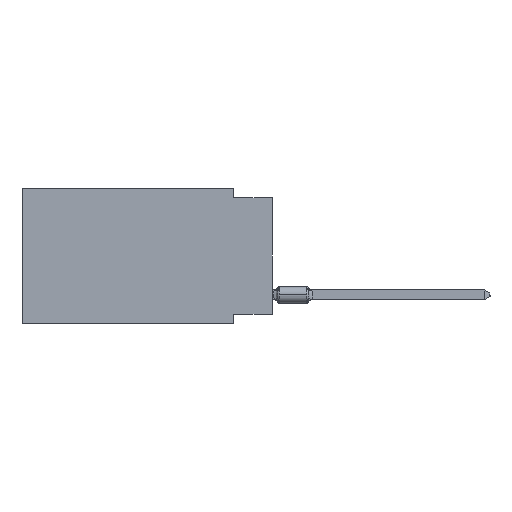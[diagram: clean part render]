
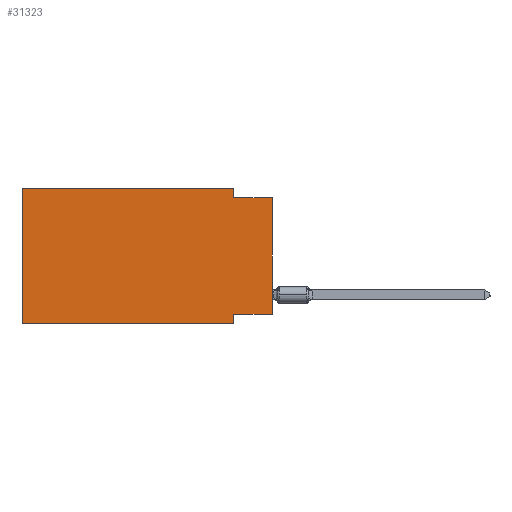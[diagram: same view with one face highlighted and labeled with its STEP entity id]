
A CAD part, left-side view. The second image highlights one B-rep face of the part: STEP entity #31323.
In plain terms, the highlighted planar face has unit normal (-1, 0, 0).
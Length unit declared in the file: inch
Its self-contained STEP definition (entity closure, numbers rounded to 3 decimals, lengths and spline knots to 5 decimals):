
#214 = LINE ( 'NONE', #24951, #24612 ) ;
#519 = VECTOR ( 'NONE', #20973, 39.37008 ) ;
#602 = VECTOR ( 'NONE', #39608, 39.37008 ) ;
#625 = VERTEX_POINT ( 'NONE', #37924 ) ;
#1147 = ORIENTED_EDGE ( 'NONE', *, *, #5059, .F. ) ;
#1822 = CARTESIAN_POINT ( 'NONE',  ( 0., 0.1, 0. ) ) ;
#1832 = CARTESIAN_POINT ( 'NONE',  ( 0., 0.645, -0.35 ) ) ;
#2816 = LINE ( 'NONE', #36383, #602 ) ;
#2853 = CARTESIAN_POINT ( 'NONE',  ( 0., 0., -0.325 ) ) ;
#3285 = ORIENTED_EDGE ( 'NONE', *, *, #30769, .T. ) ;
#5000 = ORIENTED_EDGE ( 'NONE', *, *, #15550, .F. ) ;
#5059 = EDGE_CURVE ( 'NONE', #625, #25514, #17745, .T. ) ;
#5633 = LINE ( 'NONE', #12036, #6264 ) ;
#6264 = VECTOR ( 'NONE', #36581, 39.37008 ) ;
#6781 = ORIENTED_EDGE ( 'NONE', *, *, #39465, .F. ) ;
#7541 = CARTESIAN_POINT ( 'NONE',  ( 0., 0.1, 0. ) ) ;
#7728 = DIRECTION ( 'NONE',  ( 0., -1., 0. ) ) ;
#7756 = CARTESIAN_POINT ( 'NONE',  ( 0., 0., -0.025 ) ) ;
#7968 = VECTOR ( 'NONE', #17562, 39.37008 ) ;
#9102 = EDGE_CURVE ( 'NONE', #15400, #625, #14931, .T. ) ;
#9304 = CARTESIAN_POINT ( 'NONE',  ( 0., 0.1, -0.35 ) ) ;
#10879 = AXIS2_PLACEMENT_3D ( 'NONE', #29014, #20142, #32430 ) ;
#11388 = VERTEX_POINT ( 'NONE', #15089 ) ;
#11724 = CARTESIAN_POINT ( 'NONE',  ( 0., 0., -0.325 ) ) ;
#12036 = CARTESIAN_POINT ( 'NONE',  ( 0., 0., -0.025 ) ) ;
#12928 = EDGE_CURVE ( 'NONE', #27492, #26486, #5633, .T. ) ;
#14931 = LINE ( 'NONE', #11724, #34206 ) ;
#15089 = CARTESIAN_POINT ( 'NONE',  ( 0., 0.645, 0. ) ) ;
#15400 = VERTEX_POINT ( 'NONE', #2853 ) ;
#15550 = EDGE_CURVE ( 'NONE', #20915, #11388, #214, .T. ) ;
#16019 = EDGE_CURVE ( 'NONE', #20915, #25514, #31487, .T. ) ;
#17562 = DIRECTION ( 'NONE',  ( 0., 0., -1. ) ) ;
#17745 = LINE ( 'NONE', #9304, #519 ) ;
#18827 = ORIENTED_EDGE ( 'NONE', *, *, #16019, .T. ) ;
#19306 = ORIENTED_EDGE ( 'NONE', *, *, #9102, .F. ) ;
#20142 = DIRECTION ( 'NONE',  ( 1., 0., 0. ) ) ;
#20793 = VECTOR ( 'NONE', #7728, 39.37008 ) ;
#20915 = VERTEX_POINT ( 'NONE', #1832 ) ;
#20973 = DIRECTION ( 'NONE',  ( 0., 0., -1. ) ) ;
#23811 = ORIENTED_EDGE ( 'NONE', *, *, #12928, .F. ) ;
#23989 = DIRECTION ( 'NONE',  ( 0., 1., 0. ) ) ;
#24612 = VECTOR ( 'NONE', #34405, 39.37008 ) ;
#24662 = EDGE_CURVE ( 'NONE', #33475, #27492, #38302, .T. ) ;
#24951 = CARTESIAN_POINT ( 'NONE',  ( 0., 0.645, 0. ) ) ;
#25514 = VERTEX_POINT ( 'NONE', #34239 ) ;
#25995 = FACE_OUTER_BOUND ( 'NONE', #28572, .T. ) ;
#26486 = VERTEX_POINT ( 'NONE', #7756 ) ;
#27492 = VERTEX_POINT ( 'NONE', #32081 ) ;
#28572 = EDGE_LOOP ( 'NONE', ( #3285, #23811, #32847, #6781, #5000, #18827, #1147, #19306 ) ) ;
#29014 = CARTESIAN_POINT ( 'NONE',  ( 0., 0.645, 0. ) ) ;
#30682 = LINE ( 'NONE', #33100, #31640 ) ;
#30769 = EDGE_CURVE ( 'NONE', #15400, #26486, #2816, .T. ) ;
#31323 = ADVANCED_FACE ( 'NONE', ( #25995 ), #38864, .F. ) ;
#31487 = LINE ( 'NONE', #32264, #20793 ) ;
#31640 = VECTOR ( 'NONE', #39325, 39.37008 ) ;
#32081 = CARTESIAN_POINT ( 'NONE',  ( 0., 0.1, -0.025 ) ) ;
#32264 = CARTESIAN_POINT ( 'NONE',  ( 0., 0.645, -0.35 ) ) ;
#32430 = DIRECTION ( 'NONE',  ( 0., 0., -1. ) ) ;
#32847 = ORIENTED_EDGE ( 'NONE', *, *, #24662, .F. ) ;
#33100 = CARTESIAN_POINT ( 'NONE',  ( 0., 0.645, 0. ) ) ;
#33475 = VERTEX_POINT ( 'NONE', #1822 ) ;
#34206 = VECTOR ( 'NONE', #23989, 39.37008 ) ;
#34239 = CARTESIAN_POINT ( 'NONE',  ( 0., 0.1, -0.35 ) ) ;
#34405 = DIRECTION ( 'NONE',  ( 0., 0., 1. ) ) ;
#36383 = CARTESIAN_POINT ( 'NONE',  ( 0., 0., 0. ) ) ;
#36581 = DIRECTION ( 'NONE',  ( 0., -1., 0. ) ) ;
#37924 = CARTESIAN_POINT ( 'NONE',  ( 0., 0.1, -0.325 ) ) ;
#38302 = LINE ( 'NONE', #7541, #7968 ) ;
#38864 = PLANE ( 'NONE',  #10879 ) ;
#39325 = DIRECTION ( 'NONE',  ( 0., -1., 0. ) ) ;
#39465 = EDGE_CURVE ( 'NONE', #11388, #33475, #30682, .T. ) ;
#39608 = DIRECTION ( 'NONE',  ( 0., 0., 1. ) ) ;
